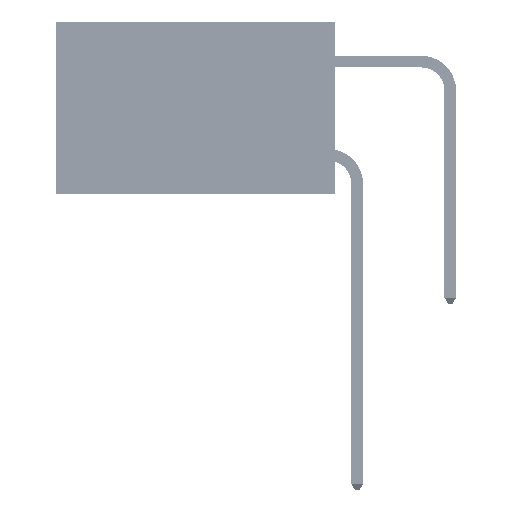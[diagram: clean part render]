
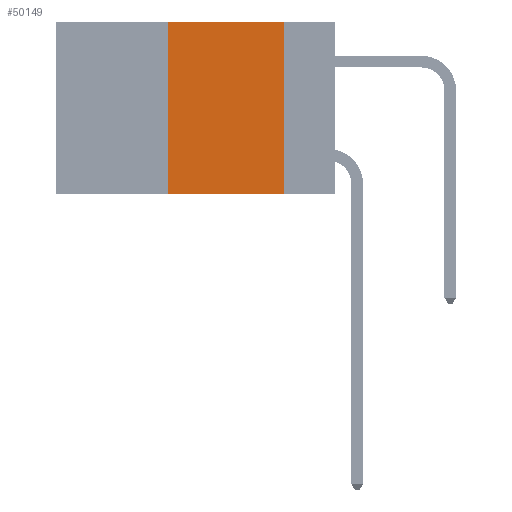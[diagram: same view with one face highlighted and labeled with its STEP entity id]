
A CAD part, left-side view. The second image highlights one B-rep face of the part: STEP entity #50149.
In plain terms, the highlighted planar face has unit normal (-1, 0, 0).
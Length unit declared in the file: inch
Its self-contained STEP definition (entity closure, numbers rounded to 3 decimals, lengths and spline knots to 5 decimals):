
#185 = DIRECTION ( 'NONE',  ( 0., -1., 0. ) ) ;
#259 = EDGE_CURVE ( 'NONE', #25293, #27325, #30265, .T. ) ;
#960 = CARTESIAN_POINT ( 'NONE',  ( 0., 0.11, 0. ) ) ;
#3438 = EDGE_LOOP ( 'NONE', ( #51797, #7718, #34312, #5634 ) ) ;
#4100 = CARTESIAN_POINT ( 'NONE',  ( 0., 0.36, -0.37 ) ) ;
#5154 = CARTESIAN_POINT ( 'NONE',  ( 0., 0.6, 0. ) ) ;
#5634 = ORIENTED_EDGE ( 'NONE', *, *, #20382, .T. ) ;
#6478 = EDGE_CURVE ( 'NONE', #27325, #17085, #12637, .T. ) ;
#6725 = PLANE ( 'NONE',  #11884 ) ;
#6776 = DIRECTION ( 'NONE',  ( 0., 0., 1. ) ) ;
#7718 = ORIENTED_EDGE ( 'NONE', *, *, #6478, .F. ) ;
#11884 = AXIS2_PLACEMENT_3D ( 'NONE', #35143, #43293, #26747 ) ;
#12637 = LINE ( 'NONE', #5154, #34400 ) ;
#13087 = FACE_OUTER_BOUND ( 'NONE', #3438, .T. ) ;
#16145 = VECTOR ( 'NONE', #37886, 39.37008 ) ;
#16728 = CARTESIAN_POINT ( 'NONE',  ( 0., 0.11, 0. ) ) ;
#17085 = VERTEX_POINT ( 'NONE', #16728 ) ;
#17218 = DIRECTION ( 'NONE',  ( 0., -1., 0. ) ) ;
#20382 = EDGE_CURVE ( 'NONE', #25293, #48033, #50741, .T. ) ;
#25293 = VERTEX_POINT ( 'NONE', #4100 ) ;
#26747 = DIRECTION ( 'NONE',  ( 0., 0., -1. ) ) ;
#27325 = VERTEX_POINT ( 'NONE', #27974 ) ;
#27974 = CARTESIAN_POINT ( 'NONE',  ( 0., 0.36, 0. ) ) ;
#30265 = LINE ( 'NONE', #39589, #39807 ) ;
#34312 = ORIENTED_EDGE ( 'NONE', *, *, #259, .F. ) ;
#34400 = VECTOR ( 'NONE', #185, 39.37008 ) ;
#34466 = EDGE_CURVE ( 'NONE', #17085, #48033, #49936, .T. ) ;
#35143 = CARTESIAN_POINT ( 'NONE',  ( 0., 0.6, 0. ) ) ;
#36102 = VECTOR ( 'NONE', #17218, 39.37008 ) ;
#37886 = DIRECTION ( 'NONE',  ( 0., 0., -1. ) ) ;
#39589 = CARTESIAN_POINT ( 'NONE',  ( 0., 0.36, 0. ) ) ;
#39807 = VECTOR ( 'NONE', #6776, 39.37008 ) ;
#43293 = DIRECTION ( 'NONE',  ( 1., 0., 0. ) ) ;
#48033 = VERTEX_POINT ( 'NONE', #49418 ) ;
#49418 = CARTESIAN_POINT ( 'NONE',  ( 0., 0.11, -0.37 ) ) ;
#49936 = LINE ( 'NONE', #960, #16145 ) ;
#50149 = ADVANCED_FACE ( 'NONE', ( #13087 ), #6725, .F. ) ;
#50741 = LINE ( 'NONE', #52390, #36102 ) ;
#51797 = ORIENTED_EDGE ( 'NONE', *, *, #34466, .F. ) ;
#52390 = CARTESIAN_POINT ( 'NONE',  ( 0., 0.6, -0.37 ) ) ;
